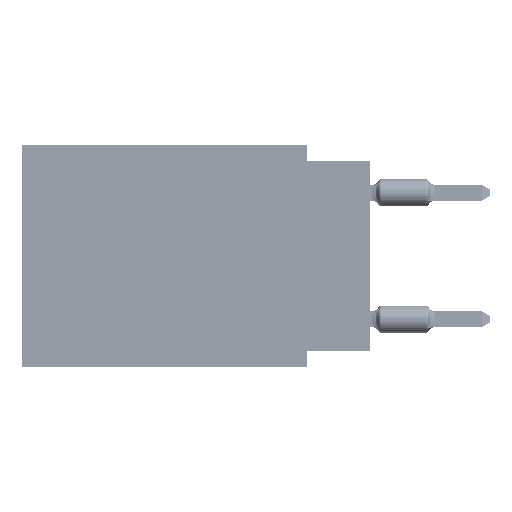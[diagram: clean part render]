
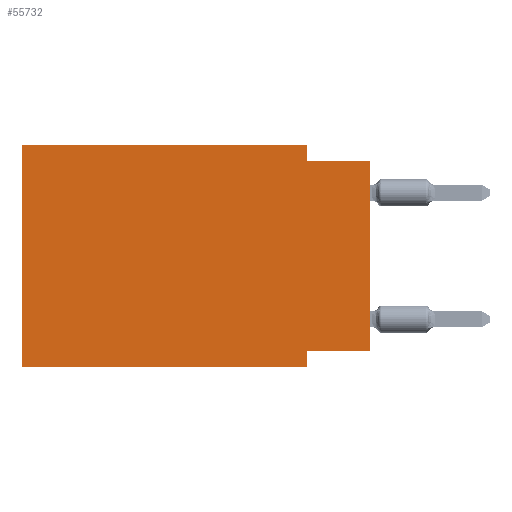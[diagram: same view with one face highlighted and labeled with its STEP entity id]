
A CAD part, left-side view. The second image highlights one B-rep face of the part: STEP entity #55732.
In plain terms, the highlighted planar face has unit normal (-1, 0, 0).
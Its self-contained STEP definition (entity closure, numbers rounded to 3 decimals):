
#569 = EDGE_CURVE ( 'NONE', #32115, #39261, #49421, .T. ) ;
#3803 = VERTEX_POINT ( 'NONE', #37709 ) ;
#4541 = EDGE_CURVE ( 'NONE', #32115, #3803, #60016, .T. ) ;
#6423 = EDGE_CURVE ( 'NONE', #58527, #12690, #68622, .T. ) ;
#7052 = CARTESIAN_POINT ( 'NONE',  ( 0., 13.97, -8.89 ) ) ;
#8418 = CARTESIAN_POINT ( 'NONE',  ( 0., 2.54, -8.255 ) ) ;
#9019 = DIRECTION ( 'NONE',  ( 0., 0., 1. ) ) ;
#9777 = CARTESIAN_POINT ( 'NONE',  ( 0., 0., 0. ) ) ;
#11319 = VECTOR ( 'NONE', #35166, 1000. ) ;
#12296 = CARTESIAN_POINT ( 'NONE',  ( 0., 0., -8.255 ) ) ;
#12329 = EDGE_CURVE ( 'NONE', #67769, #31875, #61433, .T. ) ;
#12690 = VERTEX_POINT ( 'NONE', #55977 ) ;
#13574 = LINE ( 'NONE', #54513, #56893 ) ;
#13850 = CARTESIAN_POINT ( 'NONE',  ( 0., 13.97, -8.89 ) ) ;
#18311 = CARTESIAN_POINT ( 'NONE',  ( 0., 13.97, 0. ) ) ;
#20350 = DIRECTION ( 'NONE',  ( 0., -1., 0. ) ) ;
#23276 = VECTOR ( 'NONE', #20350, 1000. ) ;
#23659 = DIRECTION ( 'NONE',  ( 0., 0., -1. ) ) ;
#24042 = DIRECTION ( 'NONE',  ( 1., 0., 0. ) ) ;
#24951 = EDGE_LOOP ( 'NONE', ( #26641, #58382, #58045, #50286, #41113, #69687, #38602, #68229 ) ) ;
#26641 = ORIENTED_EDGE ( 'NONE', *, *, #12329, .T. ) ;
#30942 = CARTESIAN_POINT ( 'NONE',  ( 0., 13.97, 0. ) ) ;
#31875 = VERTEX_POINT ( 'NONE', #44221 ) ;
#32115 = VERTEX_POINT ( 'NONE', #7052 ) ;
#32694 = VECTOR ( 'NONE', #36025, 1000. ) ;
#35166 = DIRECTION ( 'NONE',  ( 0., 0., 1. ) ) ;
#36025 = DIRECTION ( 'NONE',  ( 0., 1., 0. ) ) ;
#37709 = CARTESIAN_POINT ( 'NONE',  ( 0., 13.97, 0. ) ) ;
#38602 = ORIENTED_EDGE ( 'NONE', *, *, #70273, .F. ) ;
#39261 = VERTEX_POINT ( 'NONE', #66101 ) ;
#40497 = FACE_OUTER_BOUND ( 'NONE', #24951, .T. ) ;
#40896 = LINE ( 'NONE', #18311, #73627 ) ;
#41113 = ORIENTED_EDGE ( 'NONE', *, *, #4541, .F. ) ;
#41628 = LINE ( 'NONE', #54253, #54724 ) ;
#43029 = DIRECTION ( 'NONE',  ( 0., 0., -1. ) ) ;
#44221 = CARTESIAN_POINT ( 'NONE',  ( 0., 0., -0.635 ) ) ;
#46785 = EDGE_CURVE ( 'NONE', #3803, #58527, #40896, .T. ) ;
#49421 = LINE ( 'NONE', #13850, #23276 ) ;
#50286 = ORIENTED_EDGE ( 'NONE', *, *, #46785, .F. ) ;
#54253 = CARTESIAN_POINT ( 'NONE',  ( 0., 0., -0.635 ) ) ;
#54513 = CARTESIAN_POINT ( 'NONE',  ( 0., 2.54, -8.89 ) ) ;
#54724 = VECTOR ( 'NONE', #59979, 1000. ) ;
#55732 = ADVANCED_FACE ( 'NONE', ( #40497 ), #64961, .F. ) ;
#55977 = CARTESIAN_POINT ( 'NONE',  ( 0., 2.54, -0.635 ) ) ;
#56489 = AXIS2_PLACEMENT_3D ( 'NONE', #71086, #24042, #23659 ) ;
#56893 = VECTOR ( 'NONE', #43029, 1000. ) ;
#58045 = ORIENTED_EDGE ( 'NONE', *, *, #6423, .F. ) ;
#58382 = ORIENTED_EDGE ( 'NONE', *, *, #72646, .F. ) ;
#58527 = VERTEX_POINT ( 'NONE', #65468 ) ;
#58687 = VERTEX_POINT ( 'NONE', #8418 ) ;
#59979 = DIRECTION ( 'NONE',  ( 0., -1., 0. ) ) ;
#60016 = LINE ( 'NONE', #30942, #11319 ) ;
#61433 = LINE ( 'NONE', #9777, #67700 ) ;
#62955 = EDGE_CURVE ( 'NONE', #67769, #58687, #64715, .T. ) ;
#64230 = DIRECTION ( 'NONE',  ( 0., -1., 0. ) ) ;
#64715 = LINE ( 'NONE', #12296, #32694 ) ;
#64961 = PLANE ( 'NONE',  #56489 ) ;
#65468 = CARTESIAN_POINT ( 'NONE',  ( 0., 2.54, 0. ) ) ;
#66101 = CARTESIAN_POINT ( 'NONE',  ( 0., 2.54, -8.89 ) ) ;
#67700 = VECTOR ( 'NONE', #9019, 1000. ) ;
#67769 = VERTEX_POINT ( 'NONE', #74116 ) ;
#68229 = ORIENTED_EDGE ( 'NONE', *, *, #62955, .F. ) ;
#68622 = LINE ( 'NONE', #69373, #70217 ) ;
#69011 = DIRECTION ( 'NONE',  ( 0., 0., -1. ) ) ;
#69373 = CARTESIAN_POINT ( 'NONE',  ( 0., 2.54, 0. ) ) ;
#69687 = ORIENTED_EDGE ( 'NONE', *, *, #569, .T. ) ;
#70217 = VECTOR ( 'NONE', #69011, 1000. ) ;
#70273 = EDGE_CURVE ( 'NONE', #58687, #39261, #13574, .T. ) ;
#71086 = CARTESIAN_POINT ( 'NONE',  ( 0., 13.97, 0. ) ) ;
#72646 = EDGE_CURVE ( 'NONE', #12690, #31875, #41628, .T. ) ;
#73627 = VECTOR ( 'NONE', #64230, 1000. ) ;
#74116 = CARTESIAN_POINT ( 'NONE',  ( 0., 0., -8.255 ) ) ;
